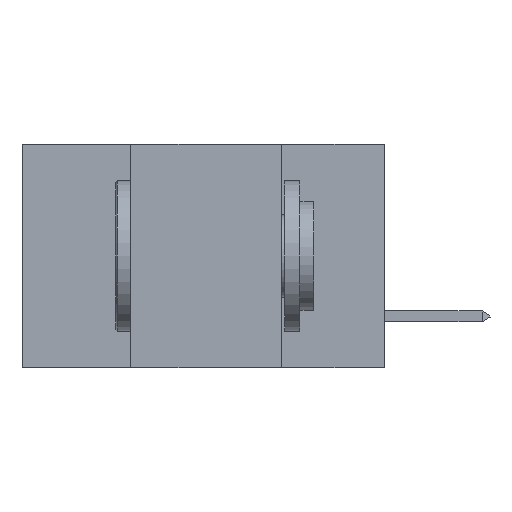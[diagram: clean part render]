
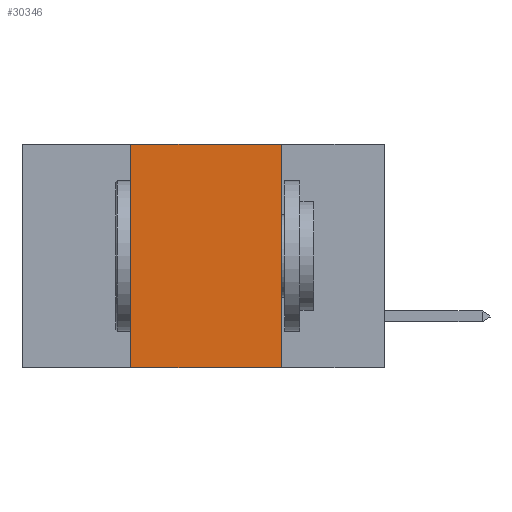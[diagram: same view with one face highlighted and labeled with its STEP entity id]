
A CAD part, left-side view. The second image highlights one B-rep face of the part: STEP entity #30346.
In plain terms, the highlighted planar face has unit normal (-1, 0, 0).
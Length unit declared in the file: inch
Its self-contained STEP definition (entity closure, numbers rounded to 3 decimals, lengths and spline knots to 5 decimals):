
#724 = DIRECTION ( 'NONE',  ( 0., 0., -1. ) ) ;
#815 = LINE ( 'NONE', #27007, #2163 ) ;
#2163 = VECTOR ( 'NONE', #32544, 39.37008 ) ;
#2621 = CARTESIAN_POINT ( 'NONE',  ( 0., 0.42, 0. ) ) ;
#4289 = EDGE_CURVE ( 'NONE', #35124, #16882, #14378, .T. ) ;
#5298 = DIRECTION ( 'NONE',  ( 1., 0., 0. ) ) ;
#5396 = DIRECTION ( 'NONE',  ( 0., 0., 1. ) ) ;
#6230 = VECTOR ( 'NONE', #5396, 39.37008 ) ;
#6265 = AXIS2_PLACEMENT_3D ( 'NONE', #32197, #5298, #32993 ) ;
#7430 = PLANE ( 'NONE',  #6265 ) ;
#8583 = CARTESIAN_POINT ( 'NONE',  ( 0., 0.17, -0.37 ) ) ;
#10004 = ORIENTED_EDGE ( 'NONE', *, *, #4289, .F. ) ;
#10922 = VERTEX_POINT ( 'NONE', #8583 ) ;
#11480 = LINE ( 'NONE', #33830, #26124 ) ;
#12770 = EDGE_CURVE ( 'NONE', #16882, #29793, #815, .T. ) ;
#13118 = ORIENTED_EDGE ( 'NONE', *, *, #19004, .F. ) ;
#13444 = CARTESIAN_POINT ( 'NONE',  ( 0., 0.42, 0. ) ) ;
#14378 = LINE ( 'NONE', #2621, #6230 ) ;
#14811 = CARTESIAN_POINT ( 'NONE',  ( 0., 0.17, 0. ) ) ;
#14869 = VECTOR ( 'NONE', #724, 39.37008 ) ;
#16882 = VERTEX_POINT ( 'NONE', #13444 ) ;
#19004 = EDGE_CURVE ( 'NONE', #29793, #10922, #23431, .T. ) ;
#23431 = LINE ( 'NONE', #14811, #14869 ) ;
#23516 = ORIENTED_EDGE ( 'NONE', *, *, #30760, .T. ) ;
#23888 = EDGE_LOOP ( 'NONE', ( #13118, #25790, #10004, #23516 ) ) ;
#25409 = DIRECTION ( 'NONE',  ( 0., -1., 0. ) ) ;
#25790 = ORIENTED_EDGE ( 'NONE', *, *, #12770, .F. ) ;
#26124 = VECTOR ( 'NONE', #25409, 39.37008 ) ;
#27007 = CARTESIAN_POINT ( 'NONE',  ( 0., 0.6, 0. ) ) ;
#28052 = FACE_OUTER_BOUND ( 'NONE', #23888, .T. ) ;
#29793 = VERTEX_POINT ( 'NONE', #30355 ) ;
#30346 = ADVANCED_FACE ( 'NONE', ( #28052 ), #7430, .F. ) ;
#30355 = CARTESIAN_POINT ( 'NONE',  ( 0., 0.17, 0. ) ) ;
#30760 = EDGE_CURVE ( 'NONE', #35124, #10922, #11480, .T. ) ;
#32195 = CARTESIAN_POINT ( 'NONE',  ( 0., 0.42, -0.37 ) ) ;
#32197 = CARTESIAN_POINT ( 'NONE',  ( 0., 0.6, 0. ) ) ;
#32544 = DIRECTION ( 'NONE',  ( 0., -1., 0. ) ) ;
#32993 = DIRECTION ( 'NONE',  ( 0., 0., -1. ) ) ;
#33830 = CARTESIAN_POINT ( 'NONE',  ( 0., 0.6, -0.37 ) ) ;
#35124 = VERTEX_POINT ( 'NONE', #32195 ) ;
